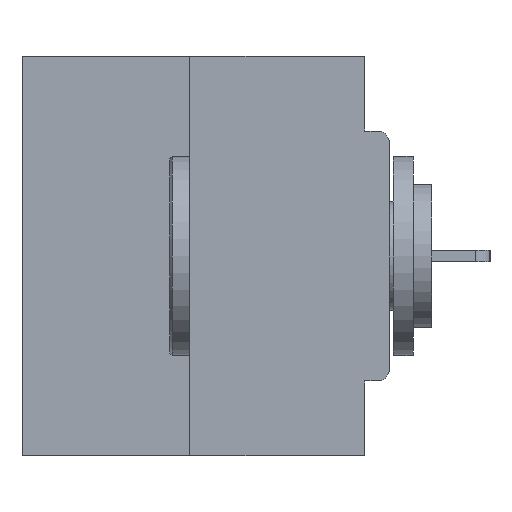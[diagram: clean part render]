
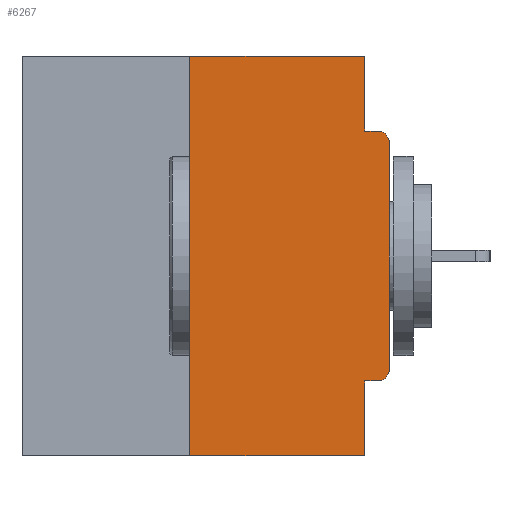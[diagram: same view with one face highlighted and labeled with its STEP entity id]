
A CAD part, left-side view. The second image highlights one B-rep face of the part: STEP entity #6267.
In plain terms, the highlighted planar face has unit normal (-1, 0, 0).
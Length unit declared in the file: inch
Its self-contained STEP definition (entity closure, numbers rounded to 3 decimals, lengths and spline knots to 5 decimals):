
#125 = ORIENTED_EDGE ( 'NONE', *, *, #19487, .F. ) ;
#1519 = EDGE_CURVE ( 'NONE', #14388, #8251, #17693, .T. ) ;
#1927 = VERTEX_POINT ( 'NONE', #35254 ) ;
#2195 = VERTEX_POINT ( 'NONE', #4088 ) ;
#2515 = CARTESIAN_POINT ( 'NONE',  ( 0., 0., -0.4065 ) ) ;
#3253 = VERTEX_POINT ( 'NONE', #17674 ) ;
#4088 = CARTESIAN_POINT ( 'NONE',  ( 0., 0.031, -0.0935 ) ) ;
#4181 = VERTEX_POINT ( 'NONE', #24704 ) ;
#4438 = LINE ( 'NONE', #4611, #34136 ) ;
#4566 = DIRECTION ( 'NONE',  ( 0., 0., 1. ) ) ;
#4611 = CARTESIAN_POINT ( 'NONE',  ( 0., 0., 0. ) ) ;
#5040 = ORIENTED_EDGE ( 'NONE', *, *, #9714, .T. ) ;
#5894 = ORIENTED_EDGE ( 'NONE', *, *, #1519, .F. ) ;
#6267 = ADVANCED_FACE ( 'NONE', ( #29931 ), #30685, .F. ) ;
#6729 = CARTESIAN_POINT ( 'NONE',  ( 0., 0.46, 0. ) ) ;
#6883 = CARTESIAN_POINT ( 'NONE',  ( 0., 0.031, -0.5 ) ) ;
#7650 = AXIS2_PLACEMENT_3D ( 'NONE', #24525, #24515, #24486 ) ;
#8251 = VERTEX_POINT ( 'NONE', #30414 ) ;
#8536 = DIRECTION ( 'NONE',  ( 0., -1., 0. ) ) ;
#8561 = EDGE_CURVE ( 'NONE', #20346, #4181, #15431, .T. ) ;
#9074 = LINE ( 'NONE', #29378, #14621 ) ;
#9126 = CARTESIAN_POINT ( 'NONE',  ( 0., 0.031, -0.4065 ) ) ;
#9321 = CARTESIAN_POINT ( 'NONE',  ( 0., 0., -0.0935 ) ) ;
#9418 = CARTESIAN_POINT ( 'NONE',  ( 0., 0.25, 0. ) ) ;
#9714 = EDGE_CURVE ( 'NONE', #30096, #20346, #4438, .T. ) ;
#9748 = CARTESIAN_POINT ( 'NONE',  ( 0., 0.015, -0.4065 ) ) ;
#9840 = ORIENTED_EDGE ( 'NONE', *, *, #14036, .T. ) ;
#9888 = CARTESIAN_POINT ( 'NONE',  ( 0., 0., -0.1085 ) ) ;
#11379 = VECTOR ( 'NONE', #11701, 39.37008 ) ;
#11701 = DIRECTION ( 'NONE',  ( 0., 0., -1. ) ) ;
#11938 = ORIENTED_EDGE ( 'NONE', *, *, #26930, .T. ) ;
#13277 = VECTOR ( 'NONE', #28285, 39.37008 ) ;
#13987 = CIRCLE ( 'NONE', #23668, 0.015 ) ;
#14036 = EDGE_CURVE ( 'NONE', #16841, #30096, #13987, .T. ) ;
#14388 = VERTEX_POINT ( 'NONE', #9418 ) ;
#14621 = VECTOR ( 'NONE', #23924, 39.37008 ) ;
#14851 = DIRECTION ( 'NONE',  ( 0., -1., 0. ) ) ;
#14953 = VERTEX_POINT ( 'NONE', #9126 ) ;
#15431 = CIRCLE ( 'NONE', #7650, 0.015 ) ;
#16044 = LINE ( 'NONE', #2515, #22381 ) ;
#16061 = EDGE_CURVE ( 'NONE', #8251, #2195, #18567, .T. ) ;
#16526 = DIRECTION ( 'NONE',  ( -1., 0., 0. ) ) ;
#16841 = VERTEX_POINT ( 'NONE', #9748 ) ;
#17521 = LINE ( 'NONE', #30987, #31824 ) ;
#17674 = CARTESIAN_POINT ( 'NONE',  ( 0., 0.25, -0.5 ) ) ;
#17693 = LINE ( 'NONE', #6729, #31177 ) ;
#17873 = EDGE_CURVE ( 'NONE', #14953, #1927, #29891, .T. ) ;
#18567 = LINE ( 'NONE', #27915, #11379 ) ;
#19487 = EDGE_CURVE ( 'NONE', #2195, #4181, #33926, .T. ) ;
#20346 = VERTEX_POINT ( 'NONE', #9888 ) ;
#20834 = CARTESIAN_POINT ( 'NONE',  ( 0., 0., -0.3915 ) ) ;
#21286 = ORIENTED_EDGE ( 'NONE', *, *, #8561, .T. ) ;
#21858 = VECTOR ( 'NONE', #31273, 39.37008 ) ;
#22381 = VECTOR ( 'NONE', #29881, 39.37008 ) ;
#23384 = ORIENTED_EDGE ( 'NONE', *, *, #30321, .F. ) ;
#23668 = AXIS2_PLACEMENT_3D ( 'NONE', #32617, #16526, #35325 ) ;
#23924 = DIRECTION ( 'NONE',  ( 0., 0., 1. ) ) ;
#24486 = DIRECTION ( 'NONE',  ( 0., 0., -1. ) ) ;
#24515 = DIRECTION ( 'NONE',  ( -1., 0., 0. ) ) ;
#24525 = CARTESIAN_POINT ( 'NONE',  ( 0., 0.015, -0.1085 ) ) ;
#24704 = CARTESIAN_POINT ( 'NONE',  ( 0., 0.015, -0.0935 ) ) ;
#25291 = AXIS2_PLACEMENT_3D ( 'NONE', #26868, #35300, #35093 ) ;
#25505 = ORIENTED_EDGE ( 'NONE', *, *, #16061, .F. ) ;
#26868 = CARTESIAN_POINT ( 'NONE',  ( 0., 0.46, 0. ) ) ;
#26930 = EDGE_CURVE ( 'NONE', #3253, #1927, #17521, .T. ) ;
#27579 = EDGE_LOOP ( 'NONE', ( #5894, #29289, #11938, #35125, #23384, #9840, #5040, #21286, #125, #25505 ) ) ;
#27915 = CARTESIAN_POINT ( 'NONE',  ( 0., 0.031, 0. ) ) ;
#28285 = DIRECTION ( 'NONE',  ( 0., -1., 0. ) ) ;
#29289 = ORIENTED_EDGE ( 'NONE', *, *, #32258, .F. ) ;
#29378 = CARTESIAN_POINT ( 'NONE',  ( 0., 0.25, 0. ) ) ;
#29881 = DIRECTION ( 'NONE',  ( 0., 1., 0. ) ) ;
#29891 = LINE ( 'NONE', #6883, #21858 ) ;
#29931 = FACE_OUTER_BOUND ( 'NONE', #27579, .T. ) ;
#30096 = VERTEX_POINT ( 'NONE', #20834 ) ;
#30321 = EDGE_CURVE ( 'NONE', #16841, #14953, #16044, .T. ) ;
#30414 = CARTESIAN_POINT ( 'NONE',  ( 0., 0.031, 0. ) ) ;
#30685 = PLANE ( 'NONE',  #25291 ) ;
#30987 = CARTESIAN_POINT ( 'NONE',  ( 0., 0.46, -0.5 ) ) ;
#31177 = VECTOR ( 'NONE', #8536, 39.37008 ) ;
#31273 = DIRECTION ( 'NONE',  ( 0., 0., -1. ) ) ;
#31824 = VECTOR ( 'NONE', #14851, 39.37008 ) ;
#32258 = EDGE_CURVE ( 'NONE', #3253, #14388, #9074, .T. ) ;
#32617 = CARTESIAN_POINT ( 'NONE',  ( 0., 0.015, -0.3915 ) ) ;
#33926 = LINE ( 'NONE', #9321, #13277 ) ;
#34136 = VECTOR ( 'NONE', #4566, 39.37008 ) ;
#35093 = DIRECTION ( 'NONE',  ( 0., 0., -1. ) ) ;
#35125 = ORIENTED_EDGE ( 'NONE', *, *, #17873, .F. ) ;
#35254 = CARTESIAN_POINT ( 'NONE',  ( 0., 0.031, -0.5 ) ) ;
#35300 = DIRECTION ( 'NONE',  ( 1., 0., 0. ) ) ;
#35325 = DIRECTION ( 'NONE',  ( 0., 0., -1. ) ) ;
